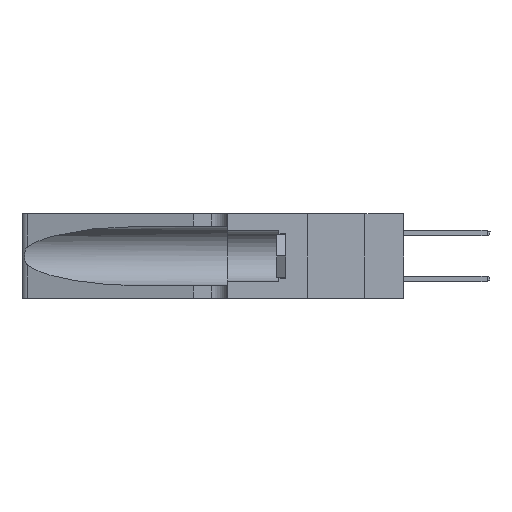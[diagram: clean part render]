
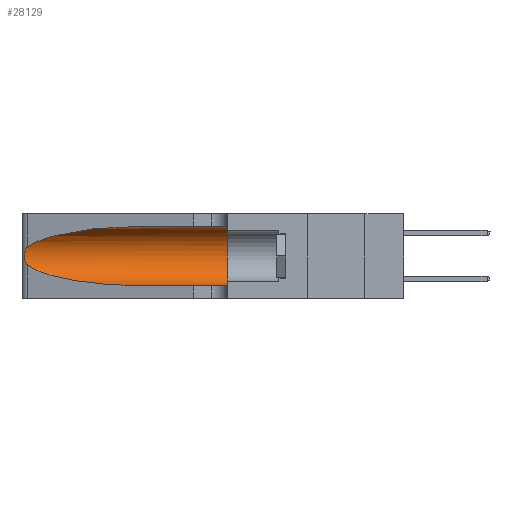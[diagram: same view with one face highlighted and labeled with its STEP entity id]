
A CAD part, left-side view. The second image highlights one B-rep face of the part: STEP entity #28129.
In plain terms, the highlighted cylindrical face has radius 3.308 mm (diameter 6.617 mm), a partial arc.
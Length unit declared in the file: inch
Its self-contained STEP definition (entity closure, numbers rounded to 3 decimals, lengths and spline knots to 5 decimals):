
#213 = CARTESIAN_POINT ( 'NONE',  ( 0.18966, 0.96281, 0.31525 ) ) ;
#483 = EDGE_CURVE ( 'NONE', #27925, #5111, #25050, .T. ) ;
#714 = DIRECTION ( 'NONE',  ( 0., -1., 0. ) ) ;
#1506 = DIRECTION ( 'NONE',  ( 0., 0., 1. ) ) ;
#2387 = CARTESIAN_POINT ( 'NONE',  ( 0.25639, 1.23184, 0.21858 ) ) ;
#2561 = CARTESIAN_POINT ( 'NONE',  ( 0.1305, 0.35, 0.05475 ) ) ;
#2926 = CARTESIAN_POINT ( 'NONE',  ( 0.26075, 1.23896, 0.178 ) ) ;
#3055 = CARTESIAN_POINT ( 'NONE',  ( 0.25555, 1.22993, 0.14849 ) ) ;
#3113 = VECTOR ( 'NONE', #39090, 39.37008 ) ;
#3327 = EDGE_CURVE ( 'NONE', #18771, #39798, #24014, .T. ) ;
#4108 = CARTESIAN_POINT ( 'NONE',  ( 0.1305, 0.35, 0.31525 ) ) ;
#4481 = CARTESIAN_POINT ( 'NONE',  ( 0.1305, 1.61858, 0.31525 ) ) ;
#5111 = VERTEX_POINT ( 'NONE', #13123 ) ;
#5316 = ORIENTED_EDGE ( 'NONE', *, *, #483, .T. ) ;
#6077 = CARTESIAN_POINT ( 'NONE',  ( 0.26017, 1.23833, 0.17102 ) ) ;
#6581 = ORIENTED_EDGE ( 'NONE', *, *, #3327, .F. ) ;
#7209 = DIRECTION ( 'NONE',  ( 0., 0., -1. ) ) ;
#8218 = VERTEX_POINT ( 'NONE', #33448 ) ;
#8288 = VERTEX_POINT ( 'NONE', #2561 ) ;
#8842 = CARTESIAN_POINT ( 'NONE',  ( 0.1305, 0.72297, 0.05475 ) ) ;
#9302 = CARTESIAN_POINT ( 'NONE',  ( 0.25856, 1.23593, 0.16098 ) ) ;
#11506 = ORIENTED_EDGE ( 'NONE', *, *, #20160, .T. ) ;
#11718 = EDGE_LOOP ( 'NONE', ( #29877, #25901, #5316, #11506, #31620, #6581 ) ) ;
#12177 = CARTESIAN_POINT ( 'NONE',  ( 0.18966, 0.96281, 0.05475 ) ) ;
#13123 = CARTESIAN_POINT ( 'NONE',  ( 0.1305, 0.72297, 0.05475 ) ) ;
#13254 = CARTESIAN_POINT ( 'NONE',  ( 0.25487, 1.22718, 0.22369 ) ) ;
#15258 = AXIS2_PLACEMENT_3D ( 'NONE', #29341, #714, #7209 ) ;
#15364 = VECTOR ( 'NONE', #35007, 39.37008 ) ;
#16063 = B_SPLINE_CURVE_WITH_KNOTS ( 'NONE', 3,
 ( #27804, #34494, #2387, #37690, #25005, #41000, #21953, #2926, #6077, #9302, #31552, #22228, #3055, #38342 ),
 .UNSPECIFIED., .F., .F.,
 ( 4, 2, 2, 2, 2, 2, 4 ),
 ( 0., 0.00027, 0.00053, 0.00107, 0.0016, 0.00187, 0.00214 ),
 .UNSPECIFIED. ) ;
#17285 = DIRECTION ( 'NONE',  ( 0., 1., 0. ) ) ;
#18771 = VERTEX_POINT ( 'NONE', #30258 ) ;
#19813 = FACE_OUTER_BOUND ( 'NONE', #11718, .T. ) ;
#20160 = EDGE_CURVE ( 'NONE', #5111, #8288, #32279, .T. ) ;
#21953 = CARTESIAN_POINT ( 'NONE',  ( 0.26075, 1.23896, 0.19203 ) ) ;
#22021 = CARTESIAN_POINT ( 'NONE',  ( 0.2373, 1.15595, 0.08982 ) ) ;
#22228 = CARTESIAN_POINT ( 'NONE',  ( 0.25639, 1.23186, 0.15144 ) ) ;
#22737 = EDGE_CURVE ( 'NONE', #39798, #8288, #30919, .T. ) ;
#23114 = AXIS2_PLACEMENT_3D ( 'NONE', #36401, #17285, #1506 ) ;
#24014 = LINE ( 'NONE', #4481, #3113 ) ;
#24211 = EDGE_CURVE ( 'NONE', #18771, #8218, #25285, .T. ) ;
#25005 = CARTESIAN_POINT ( 'NONE',  ( 0.25854, 1.2359, 0.20912 ) ) ;
#25050 =( BOUNDED_CURVE ( )  B_SPLINE_CURVE ( 3, ( #37621, #22021, #12177, #8842 ),
 .UNSPECIFIED., .F., .T. ) 
 B_SPLINE_CURVE_WITH_KNOTS ( ( 4, 4 ),
 ( 3.44316, 4.71239 ),
 .UNSPECIFIED. ) 
 CURVE ( )  GEOMETRIC_REPRESENTATION_ITEM ( )  RATIONAL_B_SPLINE_CURVE ( ( 1., 0.87, 0.87, 1. ) ) 
 REPRESENTATION_ITEM ( '' )  );
#25285 =( BOUNDED_CURVE ( )  B_SPLINE_CURVE ( 3, ( #35103, #213, #25881, #13254 ),
 .UNSPECIFIED., .F., .F. ) 
 B_SPLINE_CURVE_WITH_KNOTS ( ( 4, 4 ),
 ( 1.5708, 2.84003 ),
 .UNSPECIFIED. ) 
 CURVE ( )  GEOMETRIC_REPRESENTATION_ITEM ( )  RATIONAL_B_SPLINE_CURVE ( ( 1., 0.87, 0.87, 1. ) ) 
 REPRESENTATION_ITEM ( '' )  );
#25881 = CARTESIAN_POINT ( 'NONE',  ( 0.2373, 1.15595, 0.28018 ) ) ;
#25901 = ORIENTED_EDGE ( 'NONE', *, *, #33741, .T. ) ;
#27804 = CARTESIAN_POINT ( 'NONE',  ( 0.25487, 1.22718, 0.22369 ) ) ;
#27925 = VERTEX_POINT ( 'NONE', #40190 ) ;
#28129 = ADVANCED_FACE ( 'NONE', ( #19813 ), #32296, .F. ) ;
#29341 = CARTESIAN_POINT ( 'NONE',  ( 0.1305, 1.61858, 0.185 ) ) ;
#29877 = ORIENTED_EDGE ( 'NONE', *, *, #24211, .T. ) ;
#30258 = CARTESIAN_POINT ( 'NONE',  ( 0.1305, 0.72297, 0.31525 ) ) ;
#30919 = CIRCLE ( 'NONE', #23114, 0.13025 ) ;
#31552 = CARTESIAN_POINT ( 'NONE',  ( 0.25789, 1.23486, 0.15765 ) ) ;
#31620 = ORIENTED_EDGE ( 'NONE', *, *, #22737, .F. ) ;
#32279 = LINE ( 'NONE', #39296, #15364 ) ;
#32296 = CYLINDRICAL_SURFACE ( 'NONE', #15258, 0.13025 ) ;
#33448 = CARTESIAN_POINT ( 'NONE',  ( 0.25487, 1.22718, 0.22369 ) ) ;
#33741 = EDGE_CURVE ( 'NONE', #8218, #27925, #16063, .T. ) ;
#34494 = CARTESIAN_POINT ( 'NONE',  ( 0.25555, 1.22994, 0.2215 ) ) ;
#35007 = DIRECTION ( 'NONE',  ( 0., -1., 0. ) ) ;
#35103 = CARTESIAN_POINT ( 'NONE',  ( 0.1305, 0.72297, 0.31525 ) ) ;
#36401 = CARTESIAN_POINT ( 'NONE',  ( 0.1305, 0.35, 0.185 ) ) ;
#37621 = CARTESIAN_POINT ( 'NONE',  ( 0.25487, 1.22718, 0.14631 ) ) ;
#37690 = CARTESIAN_POINT ( 'NONE',  ( 0.25787, 1.23484, 0.2124 ) ) ;
#38342 = CARTESIAN_POINT ( 'NONE',  ( 0.25487, 1.22718, 0.14631 ) ) ;
#39090 = DIRECTION ( 'NONE',  ( 0., -1., 0. ) ) ;
#39296 = CARTESIAN_POINT ( 'NONE',  ( 0.1305, 1.61858, 0.05475 ) ) ;
#39798 = VERTEX_POINT ( 'NONE', #4108 ) ;
#40190 = CARTESIAN_POINT ( 'NONE',  ( 0.25487, 1.22718, 0.14631 ) ) ;
#41000 = CARTESIAN_POINT ( 'NONE',  ( 0.26018, 1.23835, 0.19895 ) ) ;
